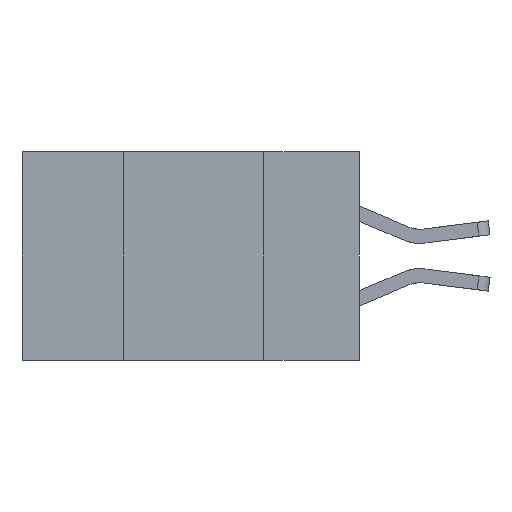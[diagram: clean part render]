
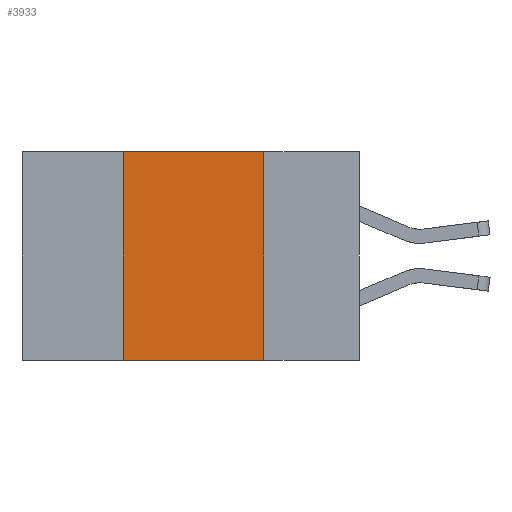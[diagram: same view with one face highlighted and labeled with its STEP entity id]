
A CAD part, left-side view. The second image highlights one B-rep face of the part: STEP entity #3933.
In plain terms, the highlighted planar face has unit normal (-1, 0, 0).
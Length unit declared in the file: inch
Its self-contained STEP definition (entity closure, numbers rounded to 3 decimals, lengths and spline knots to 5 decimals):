
#137 = DIRECTION ( 'NONE',  ( 0., -1., 0. ) ) ;
#173 = VECTOR ( 'NONE', #137, 39.37008 ) ;
#692 = CARTESIAN_POINT ( 'NONE',  ( 0., 0.6, 0. ) ) ;
#843 = CARTESIAN_POINT ( 'NONE',  ( 0., 0.17, 0. ) ) ;
#893 = DIRECTION ( 'NONE',  ( 0., -1., 0. ) ) ;
#2001 = CARTESIAN_POINT ( 'NONE',  ( 0., 0.42, 0. ) ) ;
#2298 = LINE ( 'NONE', #8888, #13742 ) ;
#2445 = VERTEX_POINT ( 'NONE', #10726 ) ;
#3040 = VECTOR ( 'NONE', #8766, 39.37008 ) ;
#3271 = EDGE_CURVE ( 'NONE', #6244, #2445, #3754, .T. ) ;
#3308 = LINE ( 'NONE', #10337, #173 ) ;
#3754 = LINE ( 'NONE', #2001, #3040 ) ;
#3933 = ADVANCED_FACE ( 'NONE', ( #12286 ), #14107, .F. ) ;
#3990 = VERTEX_POINT ( 'NONE', #843 ) ;
#4039 = EDGE_CURVE ( 'NONE', #6244, #5098, #2298, .T. ) ;
#4340 = DIRECTION ( 'NONE',  ( 0., 0., -1. ) ) ;
#4765 = CARTESIAN_POINT ( 'NONE',  ( 0., 0.42, -0.37 ) ) ;
#5098 = VERTEX_POINT ( 'NONE', #14032 ) ;
#5419 = DIRECTION ( 'NONE',  ( 0., 0., -1. ) ) ;
#6244 = VERTEX_POINT ( 'NONE', #4765 ) ;
#7515 = ORIENTED_EDGE ( 'NONE', *, *, #10673, .F. ) ;
#7756 = VECTOR ( 'NONE', #4340, 39.37008 ) ;
#7878 = ORIENTED_EDGE ( 'NONE', *, *, #3271, .F. ) ;
#8071 = EDGE_LOOP ( 'NONE', ( #10184, #7515, #7878, #10753 ) ) ;
#8766 = DIRECTION ( 'NONE',  ( 0., 0., 1. ) ) ;
#8888 = CARTESIAN_POINT ( 'NONE',  ( 0., 0.6, -0.37 ) ) ;
#10184 = ORIENTED_EDGE ( 'NONE', *, *, #11037, .F. ) ;
#10337 = CARTESIAN_POINT ( 'NONE',  ( 0., 0.6, 0. ) ) ;
#10642 = LINE ( 'NONE', #11001, #7756 ) ;
#10673 = EDGE_CURVE ( 'NONE', #2445, #3990, #3308, .T. ) ;
#10726 = CARTESIAN_POINT ( 'NONE',  ( 0., 0.42, 0. ) ) ;
#10753 = ORIENTED_EDGE ( 'NONE', *, *, #4039, .T. ) ;
#11001 = CARTESIAN_POINT ( 'NONE',  ( 0., 0.17, 0. ) ) ;
#11037 = EDGE_CURVE ( 'NONE', #3990, #5098, #10642, .T. ) ;
#11463 = AXIS2_PLACEMENT_3D ( 'NONE', #692, #12047, #5419 ) ;
#12047 = DIRECTION ( 'NONE',  ( 1., 0., 0. ) ) ;
#12286 = FACE_OUTER_BOUND ( 'NONE', #8071, .T. ) ;
#13742 = VECTOR ( 'NONE', #893, 39.37008 ) ;
#14032 = CARTESIAN_POINT ( 'NONE',  ( 0., 0.17, -0.37 ) ) ;
#14107 = PLANE ( 'NONE',  #11463 ) ;
